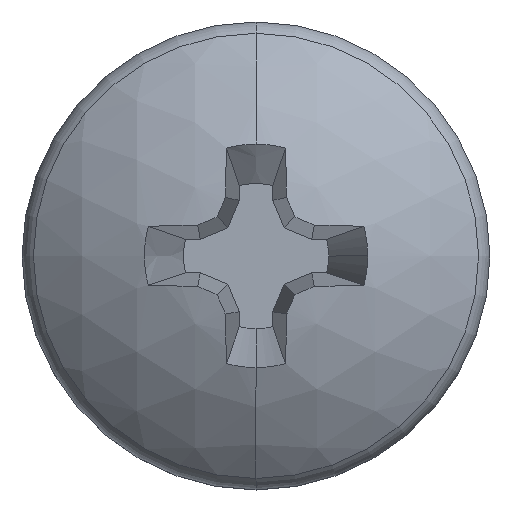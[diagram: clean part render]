
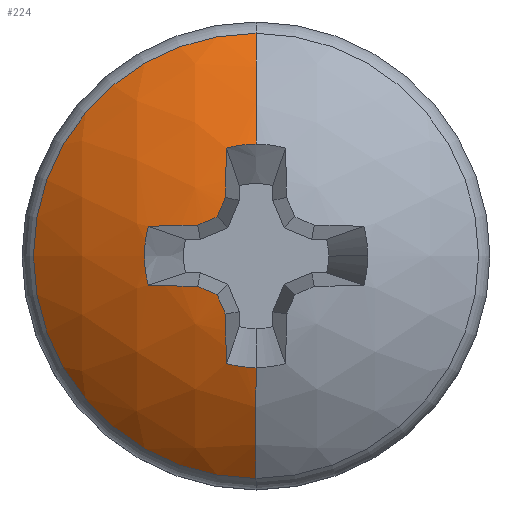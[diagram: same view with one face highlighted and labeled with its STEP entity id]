
A CAD part, top view. The second image highlights one B-rep face of the part: STEP entity #224.
In plain terms, the highlighted spherical face has radius 4.225 mm.
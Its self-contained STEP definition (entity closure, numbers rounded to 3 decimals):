
#114 = EDGE_LOOP ( 'NONE', ( #17855, #17288, #2438, #22165, #10684, #18708, #6146, #4510, #17830, #15182, #18537, #5981, #7487, #6525 ) ) ;
#141 = CARTESIAN_POINT ( 'NONE',  ( 0., 0., 48.275 ) ) ;
#224 = ADVANCED_FACE ( 'NONE', ( #13038 ), #3992, .T. ) ;
#312 = EDGE_CURVE ( 'NONE', #10230, #2171, #16548, .T. ) ;
#492 = EDGE_CURVE ( 'NONE', #12392, #25242, #4311, .T. ) ;
#525 = CIRCLE ( 'NONE', #4895, 4.225 ) ;
#556 = CARTESIAN_POINT ( 'NONE',  ( 0., -2.854, 51.39 ) ) ;
#1252 = AXIS2_PLACEMENT_3D ( 'NONE', #14741, #2380, #16820 ) ;
#1319 = AXIS2_PLACEMENT_3D ( 'NONE', #22473, #22056, #22020 ) ;
#1842 = CIRCLE ( 'NONE', #10564, 4.215 ) ;
#2171 = VERTEX_POINT ( 'NONE', #23160 ) ;
#2273 = DIRECTION ( 'NONE',  ( 0., 0., -1. ) ) ;
#2380 = DIRECTION ( 'NONE',  ( 0., 0., 1. ) ) ;
#2438 = ORIENTED_EDGE ( 'NONE', *, *, #19750, .F. ) ;
#2775 = CARTESIAN_POINT ( 'NONE',  ( -0.263, 0.109, 48.25 ) ) ;
#3095 = CIRCLE ( 'NONE', #15354, 1.433 ) ;
#3264 = VERTEX_POINT ( 'NONE', #24824 ) ;
#3992 = SPHERICAL_SURFACE ( 'NONE', #1319, 4.225 ) ;
#4063 = CARTESIAN_POINT ( 'NONE',  ( 0., 2.854, 51.39 ) ) ;
#4311 = CIRCLE ( 'NONE', #24878, 1.433 ) ;
#4510 = ORIENTED_EDGE ( 'NONE', *, *, #24922, .F. ) ;
#4605 = CARTESIAN_POINT ( 'NONE',  ( -0.393, 0.749, 52.415 ) ) ;
#4704 = VERTEX_POINT ( 'NONE', #9367 ) ;
#4868 = DIRECTION ( 'NONE',  ( 0.383, 0.924, 0. ) ) ;
#4895 = AXIS2_PLACEMENT_3D ( 'NONE', #23469, #11134, #25515 ) ;
#5397 = CARTESIAN_POINT ( 'NONE',  ( -0.109, -0.263, 48.25 ) ) ;
#5409 = EDGE_CURVE ( 'NONE', #21459, #4704, #26141, .T. ) ;
#5861 = VERTEX_POINT ( 'NONE', #4605 ) ;
#5981 = ORIENTED_EDGE ( 'NONE', *, *, #18517, .F. ) ;
#6052 = DIRECTION ( 'NONE',  ( 0.381, -0.92, 0.087 ) ) ;
#6106 = VERTEX_POINT ( 'NONE', #9565 ) ;
#6146 = ORIENTED_EDGE ( 'NONE', *, *, #10621, .F. ) ;
#6194 = VERTEX_POINT ( 'NONE', #7870 ) ;
#6525 = ORIENTED_EDGE ( 'NONE', *, *, #10782, .F. ) ;
#6789 = AXIS2_PLACEMENT_3D ( 'NONE', #20944, #8614, #23025 ) ;
#6836 = EDGE_CURVE ( 'NONE', #12831, #21459, #13879, .T. ) ;
#7487 = ORIENTED_EDGE ( 'NONE', *, *, #492, .F. ) ;
#7490 = DIRECTION ( 'NONE',  ( -0.924, 0.383, 0. ) ) ;
#7496 = CARTESIAN_POINT ( 'NONE',  ( -0.378, 1.382, 52.25 ) ) ;
#7870 = CARTESIAN_POINT ( 'NONE',  ( -0.749, -0.393, 52.415 ) ) ;
#8499 = AXIS2_PLACEMENT_3D ( 'NONE', #11972, #26312, #14020 ) ;
#8614 = DIRECTION ( 'NONE',  ( 0., -0.996, 0.087 ) ) ;
#9306 = CARTESIAN_POINT ( 'NONE',  ( 0., 0., 48.275 ) ) ;
#9364 = AXIS2_PLACEMENT_3D ( 'NONE', #141, #14632, #2273 ) ;
#9367 = CARTESIAN_POINT ( 'NONE',  ( 0., -1.433, 52.25 ) ) ;
#9565 = CARTESIAN_POINT ( 'NONE',  ( -0.499, 0.499, 52.441 ) ) ;
#9642 = CARTESIAN_POINT ( 'NONE',  ( -1.382, -0.378, 52.25 ) ) ;
#9698 = AXIS2_PLACEMENT_3D ( 'NONE', #20302, #20265, #20240 ) ;
#9742 = EDGE_CURVE ( 'NONE', #6106, #14747, #1842, .T. ) ;
#10062 = CARTESIAN_POINT ( 'NONE',  ( 0., 0., 52.25 ) ) ;
#10230 = VERTEX_POINT ( 'NONE', #20546 ) ;
#10564 = AXIS2_PLACEMENT_3D ( 'NONE', #18394, #6052, #20481 ) ;
#10621 = EDGE_CURVE ( 'NONE', #19683, #6194, #17693, .T. ) ;
#10684 = ORIENTED_EDGE ( 'NONE', *, *, #312, .F. ) ;
#10782 = EDGE_CURVE ( 'NONE', #12831, #12392, #10953, .T. ) ;
#10953 = CIRCLE ( 'NONE', #9364, 4.225 ) ;
#10960 = AXIS2_PLACEMENT_3D ( 'NONE', #5397, #19821, #7490 ) ;
#11134 = DIRECTION ( 'NONE',  ( 0.996, 0., 0.087 ) ) ;
#11388 = DIRECTION ( 'NONE',  ( 0., -1., 0. ) ) ;
#11715 = DIRECTION ( 'NONE',  ( 0.996, 0., 0.087 ) ) ;
#11880 = CARTESIAN_POINT ( 'NONE',  ( 0., 0., 52.25 ) ) ;
#11972 = CARTESIAN_POINT ( 'NONE',  ( 0., -0.03, 48.272 ) ) ;
#11987 = EDGE_CURVE ( 'NONE', #6194, #10230, #18279, .T. ) ;
#12083 = CIRCLE ( 'NONE', #12128, 4.215 ) ;
#12114 = DIRECTION ( 'NONE',  ( -1., 0., 0. ) ) ;
#12128 = AXIS2_PLACEMENT_3D ( 'NONE', #2775, #17203, #4868 ) ;
#12392 = VERTEX_POINT ( 'NONE', #20417 ) ;
#12831 = VERTEX_POINT ( 'NONE', #4063 ) ;
#13038 = FACE_OUTER_BOUND ( 'NONE', #114, .T. ) ;
#13879 = CIRCLE ( 'NONE', #1252, 2.854 ) ;
#13918 = AXIS2_PLACEMENT_3D ( 'NONE', #24051, #11715, #26067 ) ;
#13927 = DIRECTION ( 'NONE',  ( 0., 1., 0. ) ) ;
#14020 = DIRECTION ( 'NONE',  ( 0., -0.087, 0.996 ) ) ;
#14632 = DIRECTION ( 'NONE',  ( 1., 0., 0. ) ) ;
#14741 = CARTESIAN_POINT ( 'NONE',  ( 0., 0., 51.39 ) ) ;
#14747 = VERTEX_POINT ( 'NONE', #14769 ) ;
#14769 = CARTESIAN_POINT ( 'NONE',  ( -0.749, 0.393, 52.415 ) ) ;
#15182 = ORIENTED_EDGE ( 'NONE', *, *, #9742, .F. ) ;
#15354 = AXIS2_PLACEMENT_3D ( 'NONE', #11880, #26229, #13927 ) ;
#15619 = EDGE_CURVE ( 'NONE', #2171, #3264, #525, .T. ) ;
#16425 = VERTEX_POINT ( 'NONE', #17001 ) ;
#16548 = CIRCLE ( 'NONE', #9698, 4.215 ) ;
#16820 = DIRECTION ( 'NONE',  ( 0., -1., 0. ) ) ;
#17001 = CARTESIAN_POINT ( 'NONE',  ( -1.382, 0.378, 52.25 ) ) ;
#17203 = DIRECTION ( 'NONE',  ( 0.92, -0.381, 0.087 ) ) ;
#17288 = ORIENTED_EDGE ( 'NONE', *, *, #5409, .T. ) ;
#17693 = CIRCLE ( 'NONE', #8499, 4.225 ) ;
#17830 = ORIENTED_EDGE ( 'NONE', *, *, #20780, .F. ) ;
#17855 = ORIENTED_EDGE ( 'NONE', *, *, #6836, .T. ) ;
#18250 = DIRECTION ( 'NONE',  ( -1., 0., 0. ) ) ;
#18252 = CIRCLE ( 'NONE', #19040, 1.433 ) ;
#18268 = DIRECTION ( 'NONE',  ( 0., 0., 1. ) ) ;
#18279 = CIRCLE ( 'NONE', #10960, 4.215 ) ;
#18299 = CARTESIAN_POINT ( 'NONE',  ( 0., 0., 52.25 ) ) ;
#18394 = CARTESIAN_POINT ( 'NONE',  ( -0.109, 0.263, 48.25 ) ) ;
#18517 = EDGE_CURVE ( 'NONE', #25242, #5861, #26543, .T. ) ;
#18537 = ORIENTED_EDGE ( 'NONE', *, *, #21322, .F. ) ;
#18708 = ORIENTED_EDGE ( 'NONE', *, *, #11987, .F. ) ;
#19040 = AXIS2_PLACEMENT_3D ( 'NONE', #10062, #24458, #12114 ) ;
#19683 = VERTEX_POINT ( 'NONE', #9642 ) ;
#19750 = EDGE_CURVE ( 'NONE', #3264, #4704, #3095, .T. ) ;
#19821 = DIRECTION ( 'NONE',  ( 0.381, 0.92, 0.087 ) ) ;
#19833 = CIRCLE ( 'NONE', #6789, 4.225 ) ;
#20240 = DIRECTION ( 'NONE',  ( -0.383, 0.924, 0. ) ) ;
#20265 = DIRECTION ( 'NONE',  ( 0.92, 0.381, 0.087 ) ) ;
#20302 = CARTESIAN_POINT ( 'NONE',  ( -0.263, -0.109, 48.25 ) ) ;
#20417 = CARTESIAN_POINT ( 'NONE',  ( 0., 1.433, 52.25 ) ) ;
#20481 = DIRECTION ( 'NONE',  ( 0.924, 0.383, 0. ) ) ;
#20546 = CARTESIAN_POINT ( 'NONE',  ( -0.499, -0.499, 52.441 ) ) ;
#20622 = AXIS2_PLACEMENT_3D ( 'NONE', #9306, #23713, #11388 ) ;
#20780 = EDGE_CURVE ( 'NONE', #14747, #16425, #19833, .T. ) ;
#20944 = CARTESIAN_POINT ( 'NONE',  ( 0., 0.03, 48.272 ) ) ;
#21322 = EDGE_CURVE ( 'NONE', #5861, #6106, #12083, .T. ) ;
#21459 = VERTEX_POINT ( 'NONE', #556 ) ;
#22020 = DIRECTION ( 'NONE',  ( 0., 1., 0. ) ) ;
#22056 = DIRECTION ( 'NONE',  ( -1., 0., 0. ) ) ;
#22165 = ORIENTED_EDGE ( 'NONE', *, *, #15619, .F. ) ;
#22473 = CARTESIAN_POINT ( 'NONE',  ( 0., 0., 48.275 ) ) ;
#23025 = DIRECTION ( 'NONE',  ( 0., -0.087, -0.996 ) ) ;
#23160 = CARTESIAN_POINT ( 'NONE',  ( -0.393, -0.749, 52.415 ) ) ;
#23469 = CARTESIAN_POINT ( 'NONE',  ( -0.03, 0., 48.272 ) ) ;
#23713 = DIRECTION ( 'NONE',  ( -1., 0., 0. ) ) ;
#24051 = CARTESIAN_POINT ( 'NONE',  ( -0.03, 0., 48.272 ) ) ;
#24458 = DIRECTION ( 'NONE',  ( 0., 0., 1. ) ) ;
#24824 = CARTESIAN_POINT ( 'NONE',  ( -0.378, -1.382, 52.25 ) ) ;
#24878 = AXIS2_PLACEMENT_3D ( 'NONE', #18299, #18268, #18250 ) ;
#24922 = EDGE_CURVE ( 'NONE', #16425, #19683, #18252, .T. ) ;
#25242 = VERTEX_POINT ( 'NONE', #7496 ) ;
#25515 = DIRECTION ( 'NONE',  ( 0.087, 0., -0.996 ) ) ;
#26067 = DIRECTION ( 'NONE',  ( 0.087, 0., -0.996 ) ) ;
#26141 = CIRCLE ( 'NONE', #20622, 4.225 ) ;
#26229 = DIRECTION ( 'NONE',  ( 0., 0., 1. ) ) ;
#26312 = DIRECTION ( 'NONE',  ( 0., 0.996, 0.087 ) ) ;
#26543 = CIRCLE ( 'NONE', #13918, 4.225 ) ;
